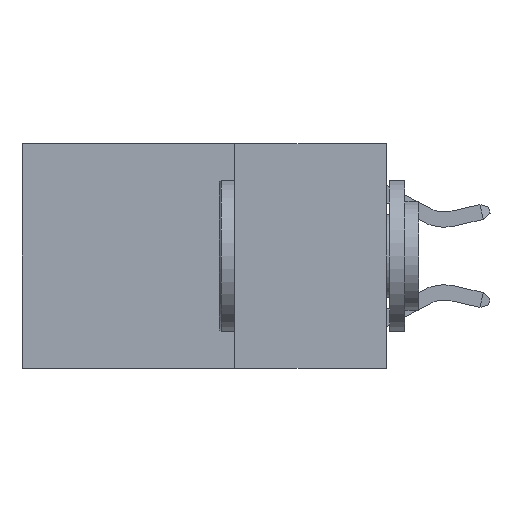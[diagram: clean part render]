
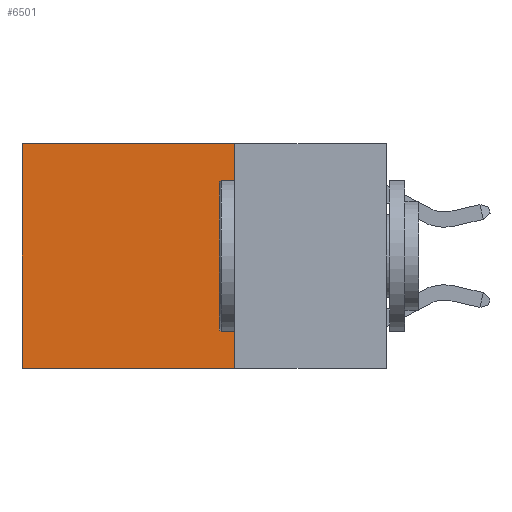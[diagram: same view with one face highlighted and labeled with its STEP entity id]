
A CAD part, left-side view. The second image highlights one B-rep face of the part: STEP entity #6501.
In plain terms, the highlighted planar face has unit normal (-1, 0, 0).
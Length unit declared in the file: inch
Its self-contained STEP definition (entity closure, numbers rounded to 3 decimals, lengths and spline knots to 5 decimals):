
#278 = DIRECTION ( 'NONE',  ( 1., 0., 0. ) ) ;
#528 = FACE_OUTER_BOUND ( 'NONE', #12878, .T. ) ;
#1286 = LINE ( 'NONE', #19729, #30031 ) ;
#2879 = DIRECTION ( 'NONE',  ( 0., 1., 0. ) ) ;
#3623 = LINE ( 'NONE', #19066, #5825 ) ;
#3869 = DIRECTION ( 'NONE',  ( 0., 0., -1. ) ) ;
#4062 = VERTEX_POINT ( 'NONE', #20237 ) ;
#5634 = CARTESIAN_POINT ( 'NONE',  ( 0.2625, 0.25, -0.37 ) ) ;
#5825 = VECTOR ( 'NONE', #9604, 39.37008 ) ;
#5979 = CARTESIAN_POINT ( 'NONE',  ( 0.2625, 0.25, 0. ) ) ;
#6273 = ORIENTED_EDGE ( 'NONE', *, *, #26391, .F. ) ;
#6501 = ADVANCED_FACE ( 'NONE', ( #528 ), #12148, .F. ) ;
#9604 = DIRECTION ( 'NONE',  ( 0., 0., -1. ) ) ;
#10875 = VERTEX_POINT ( 'NONE', #5979 ) ;
#11849 = ORIENTED_EDGE ( 'NONE', *, *, #17628, .F. ) ;
#12148 = PLANE ( 'NONE',  #21956 ) ;
#12878 = EDGE_LOOP ( 'NONE', ( #18989, #6273, #11849, #16710 ) ) ;
#14092 = VECTOR ( 'NONE', #3869, 39.37008 ) ;
#14330 = EDGE_CURVE ( 'NONE', #10875, #4062, #23037, .T. ) ;
#16147 = DIRECTION ( 'NONE',  ( 0., 1., 0. ) ) ;
#16710 = ORIENTED_EDGE ( 'NONE', *, *, #14330, .T. ) ;
#16824 = VERTEX_POINT ( 'NONE', #5634 ) ;
#16944 = DIRECTION ( 'NONE',  ( 0., 0., -1. ) ) ;
#17628 = EDGE_CURVE ( 'NONE', #10875, #16824, #3623, .T. ) ;
#17901 = EDGE_CURVE ( 'NONE', #4062, #24857, #26781, .T. ) ;
#18132 = CARTESIAN_POINT ( 'NONE',  ( 0.2625, 0.6, 0. ) ) ;
#18989 = ORIENTED_EDGE ( 'NONE', *, *, #17901, .T. ) ;
#19066 = CARTESIAN_POINT ( 'NONE',  ( 0.2625, 0.25, 0. ) ) ;
#19729 = CARTESIAN_POINT ( 'NONE',  ( 0.2625, 0.25, -0.37 ) ) ;
#20237 = CARTESIAN_POINT ( 'NONE',  ( 0.2625, 0.6, 0. ) ) ;
#20417 = VECTOR ( 'NONE', #16147, 39.37008 ) ;
#21956 = AXIS2_PLACEMENT_3D ( 'NONE', #28884, #278, #16944 ) ;
#23037 = LINE ( 'NONE', #23100, #20417 ) ;
#23100 = CARTESIAN_POINT ( 'NONE',  ( 0.2625, 0.25, 0. ) ) ;
#23894 = CARTESIAN_POINT ( 'NONE',  ( 0.2625, 0.6, -0.37 ) ) ;
#24857 = VERTEX_POINT ( 'NONE', #23894 ) ;
#26391 = EDGE_CURVE ( 'NONE', #16824, #24857, #1286, .T. ) ;
#26781 = LINE ( 'NONE', #18132, #14092 ) ;
#28884 = CARTESIAN_POINT ( 'NONE',  ( 0.2625, 0.25, 0. ) ) ;
#30031 = VECTOR ( 'NONE', #2879, 39.37008 ) ;
